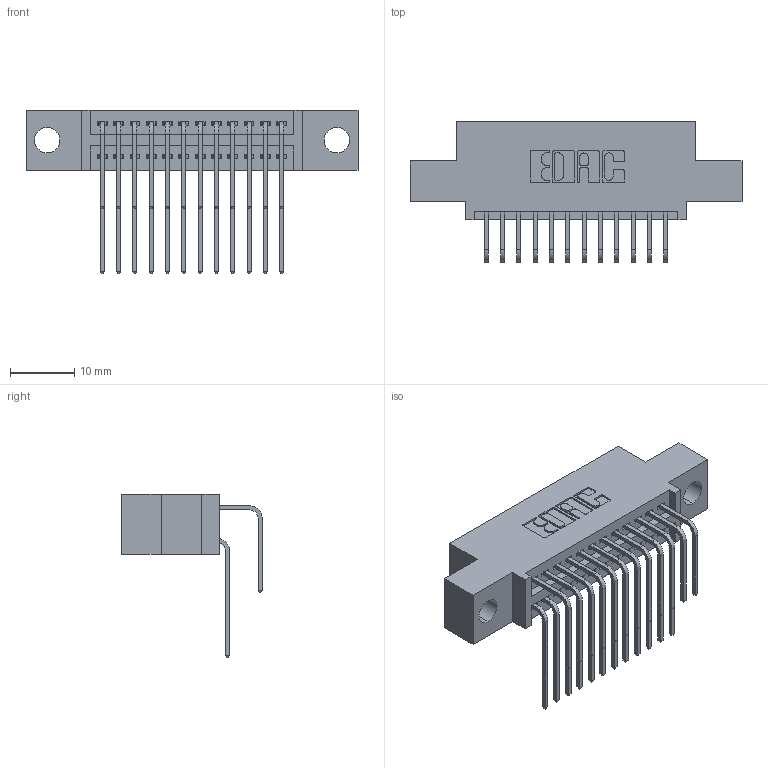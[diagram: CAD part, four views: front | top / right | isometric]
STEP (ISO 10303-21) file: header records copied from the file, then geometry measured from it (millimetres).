
FILE_DESCRIPTION (( 'STEP AP203' ), '1' );
FILE_NAME ('395-024-558-504.STEP', '2021-06-16T19:18:46', ( '' ), ( '' ), 'SwSTEP 2.0', 'SolidWorks 2020', '' );
FILE_SCHEMA (( 'CONFIG_CONTROL_DESIGN' ));
Length unit declared in the file: inch
Products named in the file (4): 395-024-558-504; 345-292-001_558 559 Tail - 1; 345 Part_0.110 Offset - 0.156 Dia-TI; 345-292-001_558 Tail - 2
Assembly tree (25 placements, depth 2):
  395-024-558-504
    345 Part_0.110 Offset - 0.156 Dia-TI
    345-292-001_558 559 Tail - 1  x12
    345-292-001_558 Tail - 2  x12
Bounding box: 51.69 x 21.83 x 25.53 mm (x, y, z)
Volume: 4701.8 mm3; surface area: 6964.5 mm2
Topology: 25 solids, 25 shells, 1392 faces, 4109 edges, 2706 vertices
Faces by surface type: plane 938, cylinder 454
Entity records: 15657 total; most frequent: CARTESIAN_POINT 2705, ORIENTED_EDGE 2586, DIRECTION 2393, EDGE_CURVE 1293, LINE 1073, VECTOR 1073, VERTEX_POINT 858, AXIS2_PLACEMENT_3D 660
